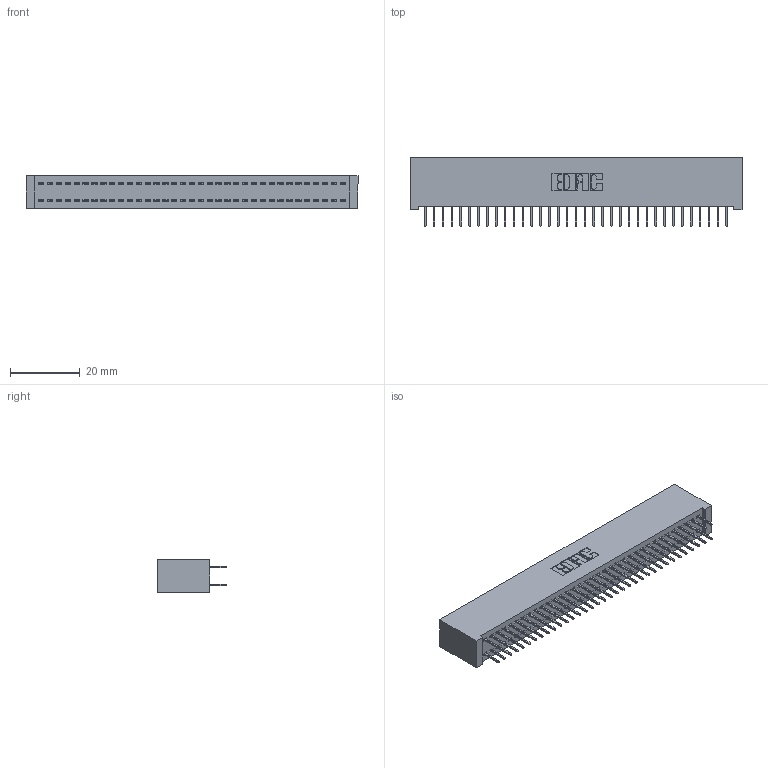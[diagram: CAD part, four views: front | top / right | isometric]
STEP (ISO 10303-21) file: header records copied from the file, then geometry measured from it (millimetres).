
FILE_DESCRIPTION (( 'STEP AP203' ), '1' );
FILE_NAME ('342-070-524-201.STEP', '2018-08-13T09:20:04', ( '' ), ( '' ), 'SwSTEP 2.0', 'SolidWorks 2016', '' );
FILE_SCHEMA (( 'CONFIG_CONTROL_DESIGN' ));
Length unit declared in the file: inch
Products named in the file (3): 342 Part_Lugless; 345-292-001_345-293-124; 342-070-524-201
Assembly tree (71 placements, depth 2):
  342-070-524-201
    342 Part_Lugless
    345-292-001_345-293-124  x70
Bounding box: 95.15 x 19.69 x 9.4 mm (x, y, z)
Volume: 8849.5 mm3; surface area: 14403 mm2
Topology: 71 solids, 71 shells, 4022 faces, 11405 edges, 7322 vertices
Faces by surface type: plane 3002, cylinder 1020
Entity records: 23087 total; most frequent: CARTESIAN_POINT 3830, ORIENTED_EDGE 3766, DIRECTION 3279, EDGE_CURVE 1883, LINE 1767, VECTOR 1767, VERTEX_POINT 1250, AXIS2_PLACEMENT_3D 756
